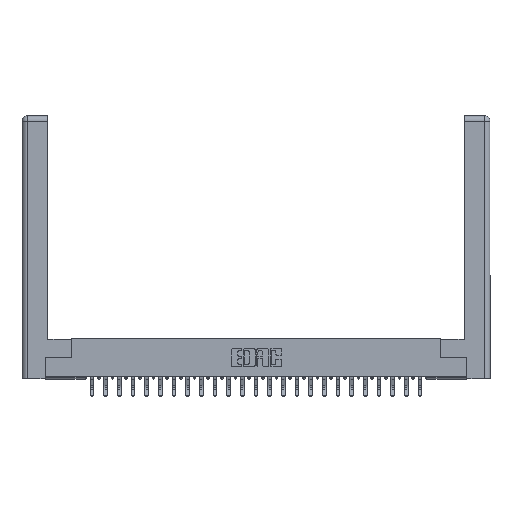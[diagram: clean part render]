
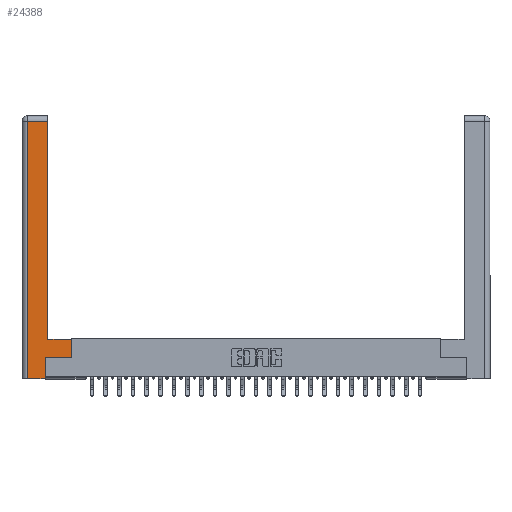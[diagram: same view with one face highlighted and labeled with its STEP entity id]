
A CAD part, top view. The second image highlights one B-rep face of the part: STEP entity #24388.
In plain terms, the highlighted planar face has unit normal (0, 0, 1).
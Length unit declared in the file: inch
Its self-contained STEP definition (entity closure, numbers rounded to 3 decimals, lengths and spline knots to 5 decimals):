
#727 = DIRECTION ( 'NONE',  ( -1., 0., 0. ) ) ;
#2098 = DIRECTION ( 'NONE',  ( 0., 1., 0. ) ) ;
#2459 = EDGE_CURVE ( 'NONE', #4313, #7667, #20606, .T. ) ;
#2776 = EDGE_CURVE ( 'NONE', #7667, #28649, #19419, .T. ) ;
#2982 = CARTESIAN_POINT ( 'NONE',  ( 0.565, 0.245, 0. ) ) ;
#3205 = CARTESIAN_POINT ( 'NONE',  ( 0.265, 0., 0. ) ) ;
#3734 = CARTESIAN_POINT ( 'NONE',  ( 0.295, 0.45, 0. ) ) ;
#4313 = VERTEX_POINT ( 'NONE', #29215 ) ;
#4364 = DIRECTION ( 'NONE',  ( -1., 0., 0. ) ) ;
#4386 = VECTOR ( 'NONE', #5664, 39.37008 ) ;
#5391 = VECTOR ( 'NONE', #5554, 39.37008 ) ;
#5554 = DIRECTION ( 'NONE',  ( 0., 1., 0. ) ) ;
#5664 = DIRECTION ( 'NONE',  ( 1., 0., 0. ) ) ;
#6155 = ORIENTED_EDGE ( 'NONE', *, *, #26922, .T. ) ;
#6652 = VECTOR ( 'NONE', #2098, 39.37008 ) ;
#7275 = VERTEX_POINT ( 'NONE', #25305 ) ;
#7525 = VERTEX_POINT ( 'NONE', #18398 ) ;
#7645 = ORIENTED_EDGE ( 'NONE', *, *, #22850, .T. ) ;
#7667 = VERTEX_POINT ( 'NONE', #25443 ) ;
#8695 = LINE ( 'NONE', #16715, #26916 ) ;
#9253 = ORIENTED_EDGE ( 'NONE', *, *, #11235, .T. ) ;
#9357 = EDGE_CURVE ( 'NONE', #23104, #7525, #26901, .T. ) ;
#9426 = DIRECTION ( 'NONE',  ( -1., 0., 0. ) ) ;
#9755 = ORIENTED_EDGE ( 'NONE', *, *, #2776, .T. ) ;
#9909 = CARTESIAN_POINT ( 'NONE',  ( 0.265, 0.245, 0. ) ) ;
#10787 = LINE ( 'NONE', #18031, #5391 ) ;
#11235 = EDGE_CURVE ( 'NONE', #28649, #23104, #12336, .T. ) ;
#11391 = FACE_OUTER_BOUND ( 'NONE', #21642, .T. ) ;
#11760 = EDGE_CURVE ( 'NONE', #24230, #31222, #10787, .T. ) ;
#12336 = LINE ( 'NONE', #26336, #18072 ) ;
#12915 = PLANE ( 'NONE',  #30454 ) ;
#14041 = VECTOR ( 'NONE', #25114, 39.37008 ) ;
#14691 = EDGE_CURVE ( 'NONE', #7525, #24230, #8695, .T. ) ;
#15578 = CARTESIAN_POINT ( 'NONE',  ( 0.265, 0.245, 0. ) ) ;
#15604 = ORIENTED_EDGE ( 'NONE', *, *, #11760, .T. ) ;
#16715 = CARTESIAN_POINT ( 'NONE',  ( 0.295, 0.45, 0. ) ) ;
#17557 = DIRECTION ( 'NONE',  ( 0., -1., 0. ) ) ;
#17570 = CARTESIAN_POINT ( 'NONE',  ( 0., 0., 0. ) ) ;
#18031 = CARTESIAN_POINT ( 'NONE',  ( 0.295, 3., 0. ) ) ;
#18072 = VECTOR ( 'NONE', #21021, 39.37008 ) ;
#18398 = CARTESIAN_POINT ( 'NONE',  ( 0.565, 0.45, 0. ) ) ;
#19336 = ORIENTED_EDGE ( 'NONE', *, *, #14691, .T. ) ;
#19419 = LINE ( 'NONE', #15578, #6652 ) ;
#19606 = VECTOR ( 'NONE', #17557, 39.37008 ) ;
#20606 = LINE ( 'NONE', #3205, #4386 ) ;
#21021 = DIRECTION ( 'NONE',  ( 1., 0., 0. ) ) ;
#21362 = LINE ( 'NONE', #31500, #27541 ) ;
#21642 = EDGE_LOOP ( 'NONE', ( #15604, #6155, #7645, #28121, #9755, #9253, #30619, #19336 ) ) ;
#22595 = CARTESIAN_POINT ( 'NONE',  ( 0.565, 0.45, 0. ) ) ;
#22850 = EDGE_CURVE ( 'NONE', #7275, #4313, #30475, .T. ) ;
#23104 = VERTEX_POINT ( 'NONE', #2982 ) ;
#24230 = VERTEX_POINT ( 'NONE', #3734 ) ;
#24388 = ADVANCED_FACE ( 'NONE', ( #11391 ), #12915, .F. ) ;
#24987 = DIRECTION ( 'NONE',  ( 0., 0., -1. ) ) ;
#25114 = DIRECTION ( 'NONE',  ( 0., 1., 0. ) ) ;
#25305 = CARTESIAN_POINT ( 'NONE',  ( 0.0615, 2.94, 0. ) ) ;
#25443 = CARTESIAN_POINT ( 'NONE',  ( 0.265, 0., 0. ) ) ;
#26336 = CARTESIAN_POINT ( 'NONE',  ( 0.565, 0.245, 0. ) ) ;
#26901 = LINE ( 'NONE', #22595, #14041 ) ;
#26916 = VECTOR ( 'NONE', #9426, 39.37008 ) ;
#26922 = EDGE_CURVE ( 'NONE', #31222, #7275, #21362, .T. ) ;
#27541 = VECTOR ( 'NONE', #4364, 39.37008 ) ;
#27759 = CARTESIAN_POINT ( 'NONE',  ( 0.295, 2.94, 0. ) ) ;
#28121 = ORIENTED_EDGE ( 'NONE', *, *, #2459, .T. ) ;
#28515 = CARTESIAN_POINT ( 'NONE',  ( 0.0615, 0., 0. ) ) ;
#28649 = VERTEX_POINT ( 'NONE', #9909 ) ;
#29215 = CARTESIAN_POINT ( 'NONE',  ( 0.0615, 0., 0. ) ) ;
#30454 = AXIS2_PLACEMENT_3D ( 'NONE', #17570, #24987, #727 ) ;
#30475 = LINE ( 'NONE', #28515, #19606 ) ;
#30619 = ORIENTED_EDGE ( 'NONE', *, *, #9357, .T. ) ;
#31222 = VERTEX_POINT ( 'NONE', #27759 ) ;
#31500 = CARTESIAN_POINT ( 'NONE',  ( 0.0615, 2.94, 0. ) ) ;
